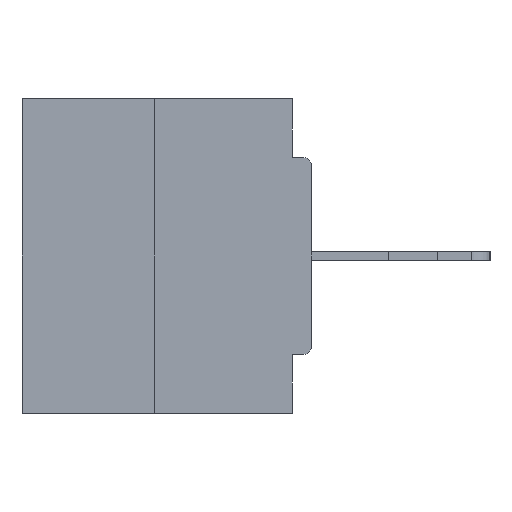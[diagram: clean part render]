
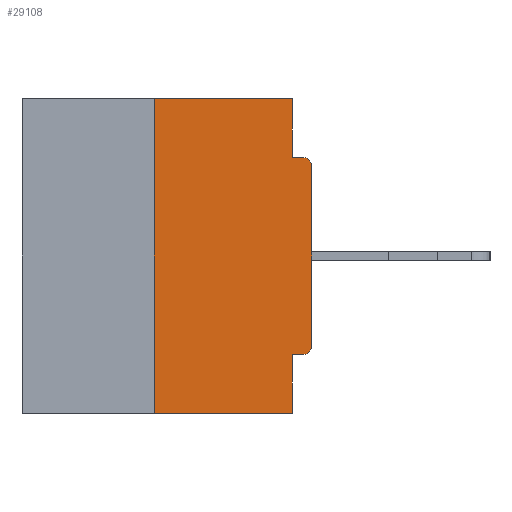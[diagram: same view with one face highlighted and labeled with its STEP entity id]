
A CAD part, left-side view. The second image highlights one B-rep face of the part: STEP entity #29108.
In plain terms, the highlighted planar face has unit normal (-1, 0, 0).
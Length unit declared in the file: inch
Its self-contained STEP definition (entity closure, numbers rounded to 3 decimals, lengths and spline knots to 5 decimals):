
#384 = LINE ( 'NONE', #33294, #25694 ) ;
#664 = DIRECTION ( 'NONE',  ( -1., 0., 0. ) ) ;
#1817 = DIRECTION ( 'NONE',  ( 0., -1., 0. ) ) ;
#1963 = ORIENTED_EDGE ( 'NONE', *, *, #14516, .T. ) ;
#2377 = PLANE ( 'NONE',  #5836 ) ;
#2518 = LINE ( 'NONE', #24439, #23280 ) ;
#2738 = ORIENTED_EDGE ( 'NONE', *, *, #34813, .T. ) ;
#2749 = EDGE_CURVE ( 'NONE', #29430, #4925, #2518, .T. ) ;
#2766 = CARTESIAN_POINT ( 'NONE',  ( 0., 0.031, -0.5 ) ) ;
#2812 = EDGE_CURVE ( 'NONE', #28060, #11843, #29653, .T. ) ;
#2976 = CARTESIAN_POINT ( 'NONE',  ( 0., 0.015, -0.3915 ) ) ;
#2977 = AXIS2_PLACEMENT_3D ( 'NONE', #2976, #14050, #25071 ) ;
#3268 = VECTOR ( 'NONE', #8069, 39.37008 ) ;
#3496 = ORIENTED_EDGE ( 'NONE', *, *, #29968, .F. ) ;
#4642 = LINE ( 'NONE', #12811, #14011 ) ;
#4925 = VERTEX_POINT ( 'NONE', #24647 ) ;
#5836 = AXIS2_PLACEMENT_3D ( 'NONE', #7821, #7641, #13439 ) ;
#6007 = DIRECTION ( 'NONE',  ( 0., 1., 0. ) ) ;
#7641 = DIRECTION ( 'NONE',  ( 1., 0., 0. ) ) ;
#7821 = CARTESIAN_POINT ( 'NONE',  ( 0., 0.46, 0. ) ) ;
#8069 = DIRECTION ( 'NONE',  ( 0., -1., 0. ) ) ;
#8312 = VERTEX_POINT ( 'NONE', #31848 ) ;
#8538 = VERTEX_POINT ( 'NONE', #21915 ) ;
#8542 = DIRECTION ( 'NONE',  ( 0., 0., 1. ) ) ;
#10175 = DIRECTION ( 'NONE',  ( 0., -1., 0. ) ) ;
#10701 = CARTESIAN_POINT ( 'NONE',  ( 0., 0., -0.0935 ) ) ;
#10924 = ORIENTED_EDGE ( 'NONE', *, *, #2749, .F. ) ;
#11843 = VERTEX_POINT ( 'NONE', #2766 ) ;
#11864 = VERTEX_POINT ( 'NONE', #12360 ) ;
#12360 = CARTESIAN_POINT ( 'NONE',  ( 0., 0.015, -0.0935 ) ) ;
#12811 = CARTESIAN_POINT ( 'NONE',  ( 0., 0.031, 0. ) ) ;
#12923 = AXIS2_PLACEMENT_3D ( 'NONE', #14444, #664, #31047 ) ;
#13439 = DIRECTION ( 'NONE',  ( 0., 0., -1. ) ) ;
#13619 = ORIENTED_EDGE ( 'NONE', *, *, #25539, .T. ) ;
#13921 = EDGE_LOOP ( 'NONE', ( #10924, #3496, #26962, #18609, #16794, #13619, #2738, #1963, #29754, #26752 ) ) ;
#13981 = CARTESIAN_POINT ( 'NONE',  ( 0., 0., -0.3915 ) ) ;
#14011 = VECTOR ( 'NONE', #31295, 39.37008 ) ;
#14050 = DIRECTION ( 'NONE',  ( -1., 0., 0. ) ) ;
#14051 = VECTOR ( 'NONE', #24268, 39.37008 ) ;
#14444 = CARTESIAN_POINT ( 'NONE',  ( 0., 0.015, -0.1085 ) ) ;
#14516 = EDGE_CURVE ( 'NONE', #8538, #11864, #31394, .T. ) ;
#14700 = EDGE_CURVE ( 'NONE', #27710, #28060, #22294, .T. ) ;
#15036 = EDGE_CURVE ( 'NONE', #8312, #11864, #18868, .T. ) ;
#16794 = ORIENTED_EDGE ( 'NONE', *, *, #14700, .F. ) ;
#18609 = ORIENTED_EDGE ( 'NONE', *, *, #2812, .F. ) ;
#18868 = LINE ( 'NONE', #10701, #20480 ) ;
#18937 = LINE ( 'NONE', #31807, #3268 ) ;
#19001 = EDGE_CURVE ( 'NONE', #31593, #11843, #18937, .T. ) ;
#20128 = CARTESIAN_POINT ( 'NONE',  ( 0., 0.031, -0.4065 ) ) ;
#20480 = VECTOR ( 'NONE', #10175, 39.37008 ) ;
#21140 = CARTESIAN_POINT ( 'NONE',  ( 0., 0.25, 0. ) ) ;
#21319 = DIRECTION ( 'NONE',  ( 0., 0., 1. ) ) ;
#21405 = FACE_OUTER_BOUND ( 'NONE', #13921, .T. ) ;
#21915 = CARTESIAN_POINT ( 'NONE',  ( 0., 0., -0.1085 ) ) ;
#22294 = LINE ( 'NONE', #33301, #27343 ) ;
#22658 = VECTOR ( 'NONE', #21319, 39.37008 ) ;
#22694 = CARTESIAN_POINT ( 'NONE',  ( 0., 0.25, -0.5 ) ) ;
#23280 = VECTOR ( 'NONE', #1817, 39.37008 ) ;
#24268 = DIRECTION ( 'NONE',  ( 0., 0., -1. ) ) ;
#24439 = CARTESIAN_POINT ( 'NONE',  ( 0., 0.46, 0. ) ) ;
#24647 = CARTESIAN_POINT ( 'NONE',  ( 0., 0.031, 0. ) ) ;
#24947 = CIRCLE ( 'NONE', #2977, 0.015 ) ;
#25071 = DIRECTION ( 'NONE',  ( 0., 0., -1. ) ) ;
#25539 = EDGE_CURVE ( 'NONE', #27710, #28009, #24947, .T. ) ;
#25694 = VECTOR ( 'NONE', #8542, 39.37008 ) ;
#25755 = CARTESIAN_POINT ( 'NONE',  ( 0., 0.015, -0.4065 ) ) ;
#26752 = ORIENTED_EDGE ( 'NONE', *, *, #30838, .F. ) ;
#26962 = ORIENTED_EDGE ( 'NONE', *, *, #19001, .T. ) ;
#26964 = CARTESIAN_POINT ( 'NONE',  ( 0., 0.031, -0.5 ) ) ;
#27091 = LINE ( 'NONE', #21140, #22658 ) ;
#27343 = VECTOR ( 'NONE', #6007, 39.37008 ) ;
#27710 = VERTEX_POINT ( 'NONE', #25755 ) ;
#28009 = VERTEX_POINT ( 'NONE', #13981 ) ;
#28060 = VERTEX_POINT ( 'NONE', #20128 ) ;
#29108 = ADVANCED_FACE ( 'NONE', ( #21405 ), #2377, .F. ) ;
#29430 = VERTEX_POINT ( 'NONE', #29826 ) ;
#29653 = LINE ( 'NONE', #26964, #14051 ) ;
#29754 = ORIENTED_EDGE ( 'NONE', *, *, #15036, .F. ) ;
#29826 = CARTESIAN_POINT ( 'NONE',  ( 0., 0.25, 0. ) ) ;
#29968 = EDGE_CURVE ( 'NONE', #31593, #29430, #27091, .T. ) ;
#30838 = EDGE_CURVE ( 'NONE', #4925, #8312, #4642, .T. ) ;
#31047 = DIRECTION ( 'NONE',  ( 0., 0., -1. ) ) ;
#31295 = DIRECTION ( 'NONE',  ( 0., 0., -1. ) ) ;
#31394 = CIRCLE ( 'NONE', #12923, 0.015 ) ;
#31593 = VERTEX_POINT ( 'NONE', #22694 ) ;
#31807 = CARTESIAN_POINT ( 'NONE',  ( 0., 0.46, -0.5 ) ) ;
#31848 = CARTESIAN_POINT ( 'NONE',  ( 0., 0.031, -0.0935 ) ) ;
#33294 = CARTESIAN_POINT ( 'NONE',  ( 0., 0., 0. ) ) ;
#33301 = CARTESIAN_POINT ( 'NONE',  ( 0., 0., -0.4065 ) ) ;
#34813 = EDGE_CURVE ( 'NONE', #28009, #8538, #384, .T. ) ;
